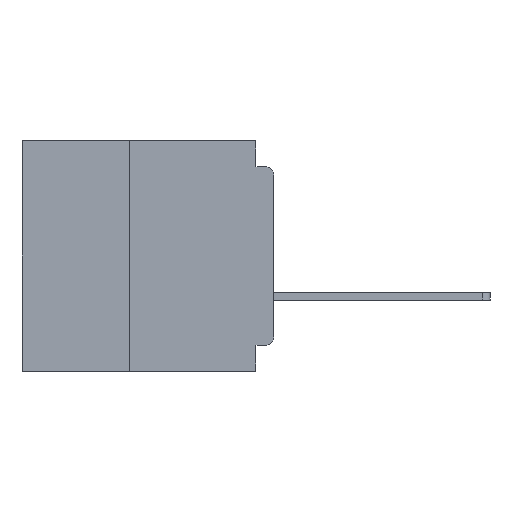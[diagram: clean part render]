
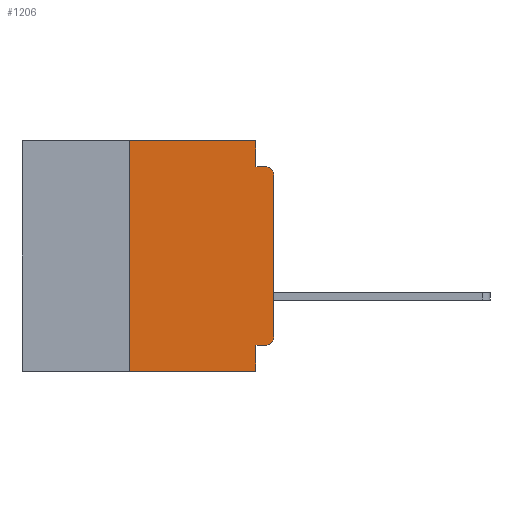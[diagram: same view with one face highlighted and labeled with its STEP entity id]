
A CAD part, left-side view. The second image highlights one B-rep face of the part: STEP entity #1206.
In plain terms, the highlighted planar face has unit normal (-1, 0, 0).
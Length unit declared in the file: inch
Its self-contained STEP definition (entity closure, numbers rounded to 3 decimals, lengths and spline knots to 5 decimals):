
#343 = VECTOR ( 'NONE', #33147, 39.37008 ) ;
#1206 = ADVANCED_FACE ( 'NONE', ( #24147 ), #6745, .F. ) ;
#1570 = EDGE_CURVE ( 'NONE', #6022, #32779, #31523, .T. ) ;
#1635 = LINE ( 'NONE', #15064, #25498 ) ;
#2876 = VECTOR ( 'NONE', #58632, 39.37008 ) ;
#3501 = VECTOR ( 'NONE', #13283, 39.37008 ) ;
#4649 = DIRECTION ( 'NONE',  ( 0., 0., -1. ) ) ;
#4908 = VERTEX_POINT ( 'NONE', #47714 ) ;
#5991 = DIRECTION ( 'NONE',  ( 1., 0., 0. ) ) ;
#6022 = VERTEX_POINT ( 'NONE', #23322 ) ;
#6745 = PLANE ( 'NONE',  #30409 ) ;
#7546 = EDGE_CURVE ( 'NONE', #22304, #56295, #15479, .T. ) ;
#8019 = EDGE_LOOP ( 'NONE', ( #33548, #46496, #55976, #16151, #16817, #9168, #23827, #46560, #25608, #23359 ) ) ;
#9168 = ORIENTED_EDGE ( 'NONE', *, *, #12965, .F. ) ;
#9176 = DIRECTION ( 'NONE',  ( -1., 0., 0. ) ) ;
#9954 = CARTESIAN_POINT ( 'NONE',  ( 0., 0., -0.34 ) ) ;
#10919 = CIRCLE ( 'NONE', #56456, 0.015 ) ;
#12965 = EDGE_CURVE ( 'NONE', #6022, #15638, #14978, .T. ) ;
#13283 = DIRECTION ( 'NONE',  ( 0., 0., 1. ) ) ;
#14978 = LINE ( 'NONE', #39283, #51214 ) ;
#15064 = CARTESIAN_POINT ( 'NONE',  ( 0., 0.031, -0.4 ) ) ;
#15479 = LINE ( 'NONE', #34975, #2876 ) ;
#15638 = VERTEX_POINT ( 'NONE', #18065 ) ;
#16151 = ORIENTED_EDGE ( 'NONE', *, *, #20011, .F. ) ;
#16297 = CARTESIAN_POINT ( 'NONE',  ( 0., 0.437, 0. ) ) ;
#16817 = ORIENTED_EDGE ( 'NONE', *, *, #53611, .F. ) ;
#16844 = VERTEX_POINT ( 'NONE', #60900 ) ;
#16925 = CARTESIAN_POINT ( 'NONE',  ( 0., 0.031, 0. ) ) ;
#18065 = CARTESIAN_POINT ( 'NONE',  ( 0., 0.25, 0. ) ) ;
#18492 = CARTESIAN_POINT ( 'NONE',  ( 0., 0.015, -0.34 ) ) ;
#19257 = CARTESIAN_POINT ( 'NONE',  ( 0., 0.031, -0.4 ) ) ;
#20011 = EDGE_CURVE ( 'NONE', #24760, #22304, #38237, .T. ) ;
#22304 = VERTEX_POINT ( 'NONE', #39368 ) ;
#23322 = CARTESIAN_POINT ( 'NONE',  ( 0., 0.25, -0.4 ) ) ;
#23326 = DIRECTION ( 'NONE',  ( 0., 0., -1. ) ) ;
#23359 = ORIENTED_EDGE ( 'NONE', *, *, #39939, .T. ) ;
#23827 = ORIENTED_EDGE ( 'NONE', *, *, #1570, .T. ) ;
#24147 = FACE_OUTER_BOUND ( 'NONE', #8019, .T. ) ;
#24760 = VERTEX_POINT ( 'NONE', #16925 ) ;
#25324 = CARTESIAN_POINT ( 'NONE',  ( 0., 0.437, 0. ) ) ;
#25498 = VECTOR ( 'NONE', #57449, 39.37008 ) ;
#25608 = ORIENTED_EDGE ( 'NONE', *, *, #32311, .F. ) ;
#25693 = DIRECTION ( 'NONE',  ( 0., -1., 0. ) ) ;
#26430 = CARTESIAN_POINT ( 'NONE',  ( 0., 0.015, -0.355 ) ) ;
#27004 = CARTESIAN_POINT ( 'NONE',  ( 0., 0.437, -0.4 ) ) ;
#27792 = EDGE_CURVE ( 'NONE', #16844, #56295, #38188, .T. ) ;
#30409 = AXIS2_PLACEMENT_3D ( 'NONE', #16297, #5991, #4649 ) ;
#31523 = LINE ( 'NONE', #27004, #52085 ) ;
#32311 = EDGE_CURVE ( 'NONE', #40271, #4908, #45692, .T. ) ;
#32779 = VERTEX_POINT ( 'NONE', #19257 ) ;
#33147 = DIRECTION ( 'NONE',  ( 0., 0., -1. ) ) ;
#33548 = ORIENTED_EDGE ( 'NONE', *, *, #48137, .T. ) ;
#34975 = CARTESIAN_POINT ( 'NONE',  ( 0., 0., -0.045 ) ) ;
#36982 = CARTESIAN_POINT ( 'NONE',  ( 0., 0., 0. ) ) ;
#37296 = CARTESIAN_POINT ( 'NONE',  ( 0., 0., -0.355 ) ) ;
#37641 = CARTESIAN_POINT ( 'NONE',  ( 0., 0.015, -0.06 ) ) ;
#38188 = CIRCLE ( 'NONE', #52253, 0.015 ) ;
#38237 = LINE ( 'NONE', #42366, #343 ) ;
#39283 = CARTESIAN_POINT ( 'NONE',  ( 0., 0.25, -0.4 ) ) ;
#39368 = CARTESIAN_POINT ( 'NONE',  ( 0., 0.031, -0.045 ) ) ;
#39939 = EDGE_CURVE ( 'NONE', #40271, #41264, #10919, .T. ) ;
#40271 = VERTEX_POINT ( 'NONE', #26430 ) ;
#41264 = VERTEX_POINT ( 'NONE', #9954 ) ;
#42313 = DIRECTION ( 'NONE',  ( 0., 0., -1. ) ) ;
#42366 = CARTESIAN_POINT ( 'NONE',  ( 0., 0.031, 0. ) ) ;
#45380 = EDGE_CURVE ( 'NONE', #4908, #32779, #1635, .T. ) ;
#45536 = LINE ( 'NONE', #25324, #56625 ) ;
#45692 = LINE ( 'NONE', #37296, #55276 ) ;
#46496 = ORIENTED_EDGE ( 'NONE', *, *, #27792, .T. ) ;
#46560 = ORIENTED_EDGE ( 'NONE', *, *, #45380, .F. ) ;
#47714 = CARTESIAN_POINT ( 'NONE',  ( 0., 0.031, -0.355 ) ) ;
#48137 = EDGE_CURVE ( 'NONE', #41264, #16844, #53824, .T. ) ;
#48711 = DIRECTION ( 'NONE',  ( 0., 0., 1. ) ) ;
#51214 = VECTOR ( 'NONE', #48711, 39.37008 ) ;
#51515 = DIRECTION ( 'NONE',  ( -1., 0., 0. ) ) ;
#52085 = VECTOR ( 'NONE', #25693, 39.37008 ) ;
#52253 = AXIS2_PLACEMENT_3D ( 'NONE', #37641, #9176, #42313 ) ;
#53297 = DIRECTION ( 'NONE',  ( 0., -1., 0. ) ) ;
#53611 = EDGE_CURVE ( 'NONE', #15638, #24760, #45536, .T. ) ;
#53824 = LINE ( 'NONE', #36982, #3501 ) ;
#54799 = CARTESIAN_POINT ( 'NONE',  ( 0., 0.015, -0.045 ) ) ;
#55276 = VECTOR ( 'NONE', #60728, 39.37008 ) ;
#55976 = ORIENTED_EDGE ( 'NONE', *, *, #7546, .F. ) ;
#56295 = VERTEX_POINT ( 'NONE', #54799 ) ;
#56456 = AXIS2_PLACEMENT_3D ( 'NONE', #18492, #51515, #23326 ) ;
#56625 = VECTOR ( 'NONE', #53297, 39.37008 ) ;
#57449 = DIRECTION ( 'NONE',  ( 0., 0., -1. ) ) ;
#58632 = DIRECTION ( 'NONE',  ( 0., -1., 0. ) ) ;
#60728 = DIRECTION ( 'NONE',  ( 0., 1., 0. ) ) ;
#60900 = CARTESIAN_POINT ( 'NONE',  ( 0., 0., -0.06 ) ) ;
